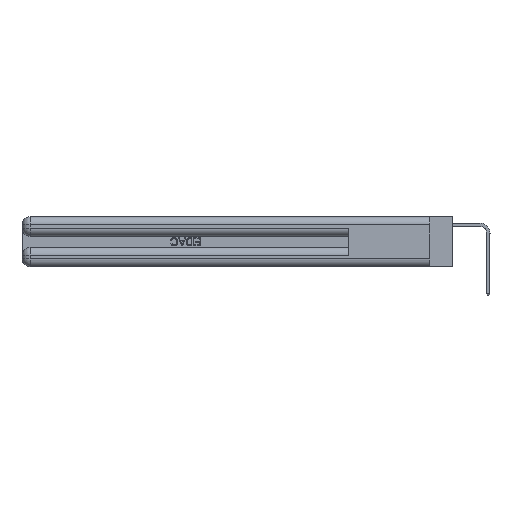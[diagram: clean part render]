
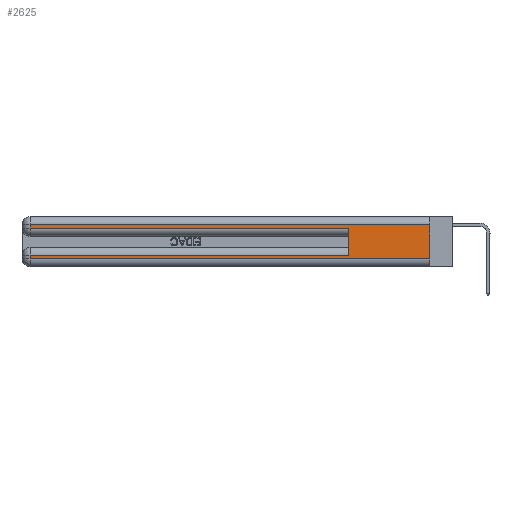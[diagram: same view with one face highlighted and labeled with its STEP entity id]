
A CAD part, left-side view. The second image highlights one B-rep face of the part: STEP entity #2625.
In plain terms, the highlighted planar face has unit normal (-1, 0, 0).
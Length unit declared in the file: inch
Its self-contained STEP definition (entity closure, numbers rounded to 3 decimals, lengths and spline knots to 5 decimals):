
#611 = VECTOR ( 'NONE', #27537, 39.37008 ) ;
#997 = VERTEX_POINT ( 'NONE', #13514 ) ;
#1291 = EDGE_CURVE ( 'NONE', #6221, #4650, #8545, .T. ) ;
#1297 = ORIENTED_EDGE ( 'NONE', *, *, #4350, .T. ) ;
#1368 = EDGE_CURVE ( 'NONE', #1910, #21023, #30894, .T. ) ;
#1910 = VERTEX_POINT ( 'NONE', #10405 ) ;
#2055 = VECTOR ( 'NONE', #30975, 39.37008 ) ;
#2625 = ADVANCED_FACE ( 'NONE', ( #19329 ), #5035, .F. ) ;
#2933 = LINE ( 'NONE', #22347, #20556 ) ;
#3407 = DIRECTION ( 'NONE',  ( 0., 0., -1. ) ) ;
#4350 = EDGE_CURVE ( 'NONE', #27471, #997, #14353, .T. ) ;
#4650 = VERTEX_POINT ( 'NONE', #5345 ) ;
#4852 = EDGE_LOOP ( 'NONE', ( #24148, #29954, #14215, #6837, #14715, #26740, #28119, #1297 ) ) ;
#4905 = LINE ( 'NONE', #21890, #29532 ) ;
#5035 = PLANE ( 'NONE',  #29337 ) ;
#5345 = CARTESIAN_POINT ( 'NONE',  ( 0., 2.94, 0.285 ) ) ;
#6221 = VERTEX_POINT ( 'NONE', #24751 ) ;
#6497 = VERTEX_POINT ( 'NONE', #18595 ) ;
#6530 = DIRECTION ( 'NONE',  ( 0., 1., 0. ) ) ;
#6837 = ORIENTED_EDGE ( 'NONE', *, *, #21828, .T. ) ;
#7129 = EDGE_CURVE ( 'NONE', #22935, #6221, #8973, .T. ) ;
#7457 = DIRECTION ( 'NONE',  ( 1., 0., 0. ) ) ;
#7474 = VECTOR ( 'NONE', #6530, 39.37008 ) ;
#7807 = VECTOR ( 'NONE', #3407, 39.37008 ) ;
#7982 = VECTOR ( 'NONE', #11461, 39.37008 ) ;
#8545 = LINE ( 'NONE', #24928, #7807 ) ;
#8973 = LINE ( 'NONE', #11265, #7474 ) ;
#10405 = CARTESIAN_POINT ( 'NONE',  ( 0., 0.6, 0.085 ) ) ;
#11265 = CARTESIAN_POINT ( 'NONE',  ( 0., 0., 0.31 ) ) ;
#11461 = DIRECTION ( 'NONE',  ( 0., -1., 0. ) ) ;
#12279 = CARTESIAN_POINT ( 'NONE',  ( 0., 2.94, 0.06 ) ) ;
#12876 = CARTESIAN_POINT ( 'NONE',  ( 0., 0.6, 0.285 ) ) ;
#13274 = CARTESIAN_POINT ( 'NONE',  ( 0., 0.6, 0.145 ) ) ;
#13372 = EDGE_CURVE ( 'NONE', #6497, #27471, #27499, .T. ) ;
#13514 = CARTESIAN_POINT ( 'NONE',  ( 0., 0., 0.06 ) ) ;
#13837 = CARTESIAN_POINT ( 'NONE',  ( 0., 0., 0.06 ) ) ;
#14215 = ORIENTED_EDGE ( 'NONE', *, *, #1291, .T. ) ;
#14353 = LINE ( 'NONE', #13837, #7982 ) ;
#14715 = ORIENTED_EDGE ( 'NONE', *, *, #1368, .F. ) ;
#15141 = DIRECTION ( 'NONE',  ( 0., 0., -1. ) ) ;
#16008 = DIRECTION ( 'NONE',  ( 0., -1., 0. ) ) ;
#16078 = EDGE_CURVE ( 'NONE', #22935, #997, #2933, .T. ) ;
#16724 = CARTESIAN_POINT ( 'NONE',  ( 0., 2.94, 0.37 ) ) ;
#18595 = CARTESIAN_POINT ( 'NONE',  ( 0., 2.94, 0.085 ) ) ;
#19329 = FACE_OUTER_BOUND ( 'NONE', #4852, .T. ) ;
#20175 = LINE ( 'NONE', #25615, #25734 ) ;
#20311 = EDGE_CURVE ( 'NONE', #1910, #6497, #4905, .T. ) ;
#20556 = VECTOR ( 'NONE', #15141, 39.37008 ) ;
#21023 = VERTEX_POINT ( 'NONE', #12876 ) ;
#21828 = EDGE_CURVE ( 'NONE', #4650, #21023, #20175, .T. ) ;
#21890 = CARTESIAN_POINT ( 'NONE',  ( 0., 0., 0.085 ) ) ;
#22347 = CARTESIAN_POINT ( 'NONE',  ( 0., 0., 0.37 ) ) ;
#22935 = VERTEX_POINT ( 'NONE', #29580 ) ;
#24062 = CARTESIAN_POINT ( 'NONE',  ( 0., 0., 0.37 ) ) ;
#24148 = ORIENTED_EDGE ( 'NONE', *, *, #16078, .F. ) ;
#24166 = DIRECTION ( 'NONE',  ( 0., 0., -1. ) ) ;
#24263 = DIRECTION ( 'NONE',  ( 0., 1., 0. ) ) ;
#24751 = CARTESIAN_POINT ( 'NONE',  ( 0., 2.94, 0.31 ) ) ;
#24928 = CARTESIAN_POINT ( 'NONE',  ( 0., 2.94, 0.37 ) ) ;
#25615 = CARTESIAN_POINT ( 'NONE',  ( 0., 0., 0.285 ) ) ;
#25734 = VECTOR ( 'NONE', #16008, 39.37008 ) ;
#26740 = ORIENTED_EDGE ( 'NONE', *, *, #20311, .T. ) ;
#27471 = VERTEX_POINT ( 'NONE', #12279 ) ;
#27499 = LINE ( 'NONE', #16724, #2055 ) ;
#27537 = DIRECTION ( 'NONE',  ( 0., 0., 1. ) ) ;
#28119 = ORIENTED_EDGE ( 'NONE', *, *, #13372, .T. ) ;
#29337 = AXIS2_PLACEMENT_3D ( 'NONE', #24062, #7457, #24166 ) ;
#29532 = VECTOR ( 'NONE', #24263, 39.37008 ) ;
#29580 = CARTESIAN_POINT ( 'NONE',  ( 0., 0., 0.31 ) ) ;
#29954 = ORIENTED_EDGE ( 'NONE', *, *, #7129, .T. ) ;
#30894 = LINE ( 'NONE', #13274, #611 ) ;
#30975 = DIRECTION ( 'NONE',  ( 0., 0., -1. ) ) ;
